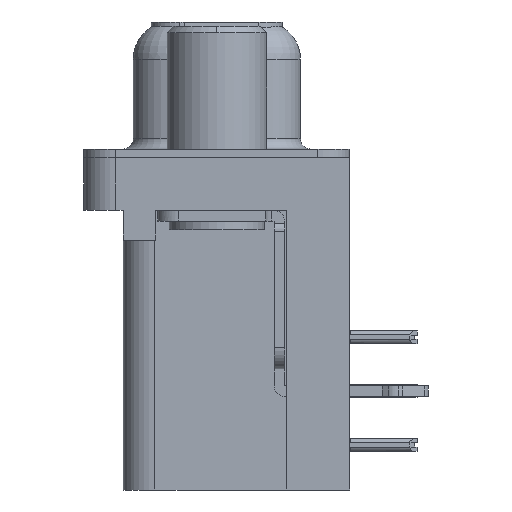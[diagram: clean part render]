
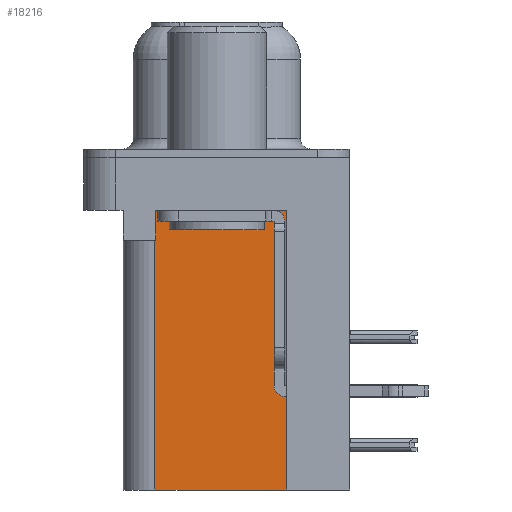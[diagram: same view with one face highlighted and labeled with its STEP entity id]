
A CAD part, left-side view. The second image highlights one B-rep face of the part: STEP entity #18216.
In plain terms, the highlighted planar face has unit normal (-1, 0, 0).
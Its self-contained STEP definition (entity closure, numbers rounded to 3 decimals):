
#198 = VERTEX_POINT ( 'NONE', #7962 ) ;
#505 = FACE_OUTER_BOUND ( 'NONE', #16836, .T. ) ;
#648 = AXIS2_PLACEMENT_3D ( 'NONE', #20266, #6025, #26168 ) ;
#1298 = CARTESIAN_POINT ( 'NONE',  ( 3.765, -3.295, -15.7 ) ) ;
#2027 = LINE ( 'NONE', #10036, #9659 ) ;
#2570 = CARTESIAN_POINT ( 'NONE',  ( 3.765, 2.925, -3.9 ) ) ;
#3116 = PLANE ( 'NONE',  #648 ) ;
#3340 = LINE ( 'NONE', #1298, #25426 ) ;
#3379 = DIRECTION ( 'NONE',  ( 0., 1., 0. ) ) ;
#6025 = DIRECTION ( 'NONE',  ( 1., 0., 0. ) ) ;
#6920 = CARTESIAN_POINT ( 'NONE',  ( 3.765, -3.295, -15.7 ) ) ;
#7962 = CARTESIAN_POINT ( 'NONE',  ( 3.765, -3.295, -2.5 ) ) ;
#8255 = ORIENTED_EDGE ( 'NONE', *, *, #37486, .T. ) ;
#9659 = VECTOR ( 'NONE', #27362, 1000. ) ;
#9962 = EDGE_CURVE ( 'NONE', #198, #29716, #18515, .T. ) ;
#10036 = CARTESIAN_POINT ( 'NONE',  ( 3.765, 2.895, -3.9 ) ) ;
#10611 = DIRECTION ( 'NONE',  ( 0., 0., 1. ) ) ;
#10946 = VECTOR ( 'NONE', #3379, 1000. ) ;
#12380 = LINE ( 'NONE', #30894, #20053 ) ;
#12485 = VECTOR ( 'NONE', #19609, 1000. ) ;
#12620 = CARTESIAN_POINT ( 'NONE',  ( 3.765, 0., -3.9 ) ) ;
#12704 = EDGE_CURVE ( 'NONE', #22801, #22341, #15223, .T. ) ;
#12824 = DIRECTION ( 'NONE',  ( 0., 0., 1. ) ) ;
#12966 = ORIENTED_EDGE ( 'NONE', *, *, #24570, .T. ) ;
#13815 = CARTESIAN_POINT ( 'NONE',  ( 3.765, -3.295, -15.7 ) ) ;
#14997 = ORIENTED_EDGE ( 'NONE', *, *, #9962, .T. ) ;
#15223 = LINE ( 'NONE', #12620, #22058 ) ;
#16836 = EDGE_LOOP ( 'NONE', ( #14997, #8255, #37586, #31087, #35967, #12966 ) ) ;
#18216 = ADVANCED_FACE ( 'NONE', ( #505 ), #3116, .F. ) ;
#18515 = LINE ( 'NONE', #20548, #10946 ) ;
#19249 = LINE ( 'NONE', #13815, #12485 ) ;
#19609 = DIRECTION ( 'NONE',  ( 0., 1., 0. ) ) ;
#20053 = VECTOR ( 'NONE', #10611, 1000. ) ;
#20240 = CARTESIAN_POINT ( 'NONE',  ( 3.765, 2.895, -2.5 ) ) ;
#20266 = CARTESIAN_POINT ( 'NONE',  ( 3.765, -3.295, -15.7 ) ) ;
#20548 = CARTESIAN_POINT ( 'NONE',  ( 3.765, -3.295, -2.5 ) ) ;
#20664 = EDGE_CURVE ( 'NONE', #35803, #27418, #19249, .T. ) ;
#21705 = CARTESIAN_POINT ( 'NONE',  ( 3.765, 2.925, -15.7 ) ) ;
#21980 = CARTESIAN_POINT ( 'NONE',  ( 3.765, 2.895, -3.9 ) ) ;
#22058 = VECTOR ( 'NONE', #27103, 1000. ) ;
#22341 = VERTEX_POINT ( 'NONE', #2570 ) ;
#22801 = VERTEX_POINT ( 'NONE', #21980 ) ;
#24570 = EDGE_CURVE ( 'NONE', #35803, #198, #3340, .T. ) ;
#25426 = VECTOR ( 'NONE', #12824, 1000. ) ;
#26168 = DIRECTION ( 'NONE',  ( 0., 0., -1. ) ) ;
#27103 = DIRECTION ( 'NONE',  ( 0., 1., 0. ) ) ;
#27362 = DIRECTION ( 'NONE',  ( 0., 0., -1. ) ) ;
#27418 = VERTEX_POINT ( 'NONE', #21705 ) ;
#29716 = VERTEX_POINT ( 'NONE', #20240 ) ;
#30894 = CARTESIAN_POINT ( 'NONE',  ( 3.765, 2.925, -15.7 ) ) ;
#31087 = ORIENTED_EDGE ( 'NONE', *, *, #31820, .F. ) ;
#31820 = EDGE_CURVE ( 'NONE', #27418, #22341, #12380, .T. ) ;
#35803 = VERTEX_POINT ( 'NONE', #6920 ) ;
#35967 = ORIENTED_EDGE ( 'NONE', *, *, #20664, .F. ) ;
#37486 = EDGE_CURVE ( 'NONE', #29716, #22801, #2027, .T. ) ;
#37586 = ORIENTED_EDGE ( 'NONE', *, *, #12704, .T. ) ;
